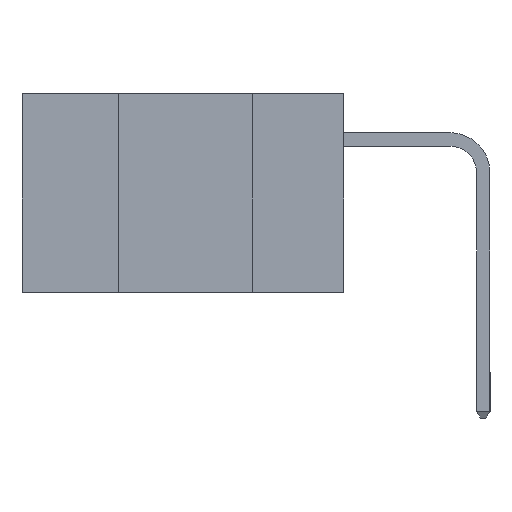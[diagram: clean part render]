
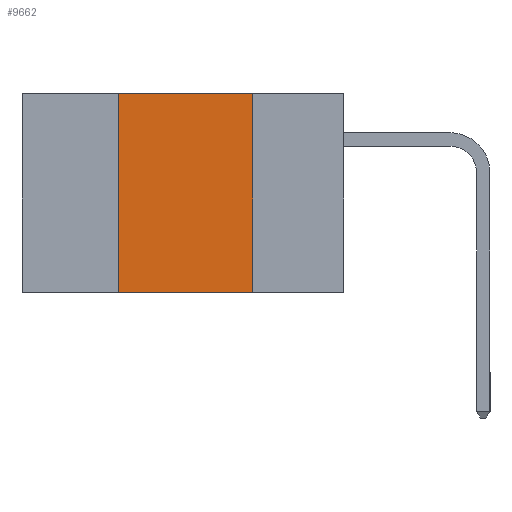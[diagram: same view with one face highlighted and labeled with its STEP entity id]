
A CAD part, left-side view. The second image highlights one B-rep face of the part: STEP entity #9662.
In plain terms, the highlighted planar face has unit normal (-1, 0, 0).
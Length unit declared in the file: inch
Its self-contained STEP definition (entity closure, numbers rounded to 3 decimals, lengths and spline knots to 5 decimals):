
#689 = LINE ( 'NONE', #21427, #14383 ) ;
#1158 = VERTEX_POINT ( 'NONE', #12335 ) ;
#1439 = VERTEX_POINT ( 'NONE', #18707 ) ;
#2466 = ORIENTED_EDGE ( 'NONE', *, *, #20753, .F. ) ;
#3195 = LINE ( 'NONE', #20866, #3905 ) ;
#3539 = ORIENTED_EDGE ( 'NONE', *, *, #6020, .F. ) ;
#3817 = VERTEX_POINT ( 'NONE', #9401 ) ;
#3905 = VECTOR ( 'NONE', #8805, 39.37008 ) ;
#4909 = LINE ( 'NONE', #9527, #7433 ) ;
#5340 = ORIENTED_EDGE ( 'NONE', *, *, #19002, .F. ) ;
#5621 = LINE ( 'NONE', #17788, #16411 ) ;
#5951 = ORIENTED_EDGE ( 'NONE', *, *, #15987, .T. ) ;
#6020 = EDGE_CURVE ( 'NONE', #1439, #1158, #689, .T. ) ;
#6101 = CARTESIAN_POINT ( 'NONE',  ( 0., 0.17, -0.37 ) ) ;
#7352 = DIRECTION ( 'NONE',  ( 0., 0., 1. ) ) ;
#7433 = VECTOR ( 'NONE', #8729, 39.37008 ) ;
#7467 = EDGE_LOOP ( 'NONE', ( #2466, #5340, #3539, #5951 ) ) ;
#8729 = DIRECTION ( 'NONE',  ( 0., -1., 0. ) ) ;
#8805 = DIRECTION ( 'NONE',  ( 0., 0., -1. ) ) ;
#8912 = FACE_OUTER_BOUND ( 'NONE', #7467, .T. ) ;
#9401 = CARTESIAN_POINT ( 'NONE',  ( 0., 0.17, 0. ) ) ;
#9527 = CARTESIAN_POINT ( 'NONE',  ( 0., 0.6, 0. ) ) ;
#9662 = ADVANCED_FACE ( 'NONE', ( #8912 ), #10275, .F. ) ;
#10275 = PLANE ( 'NONE',  #16277 ) ;
#12190 = DIRECTION ( 'NONE',  ( 1., 0., 0. ) ) ;
#12335 = CARTESIAN_POINT ( 'NONE',  ( 0., 0.42, 0. ) ) ;
#13664 = DIRECTION ( 'NONE',  ( 0., 0., -1. ) ) ;
#14383 = VECTOR ( 'NONE', #7352, 39.37008 ) ;
#15987 = EDGE_CURVE ( 'NONE', #1439, #18549, #5621, .T. ) ;
#16277 = AXIS2_PLACEMENT_3D ( 'NONE', #17054, #12190, #13664 ) ;
#16411 = VECTOR ( 'NONE', #17672, 39.37008 ) ;
#17054 = CARTESIAN_POINT ( 'NONE',  ( 0., 0.6, 0. ) ) ;
#17672 = DIRECTION ( 'NONE',  ( 0., -1., 0. ) ) ;
#17788 = CARTESIAN_POINT ( 'NONE',  ( 0., 0.6, -0.37 ) ) ;
#18549 = VERTEX_POINT ( 'NONE', #6101 ) ;
#18707 = CARTESIAN_POINT ( 'NONE',  ( 0., 0.42, -0.37 ) ) ;
#19002 = EDGE_CURVE ( 'NONE', #1158, #3817, #4909, .T. ) ;
#20753 = EDGE_CURVE ( 'NONE', #3817, #18549, #3195, .T. ) ;
#20866 = CARTESIAN_POINT ( 'NONE',  ( 0., 0.17, -0.37 ) ) ;
#21427 = CARTESIAN_POINT ( 'NONE',  ( 0., 0.42, -0.37 ) ) ;
